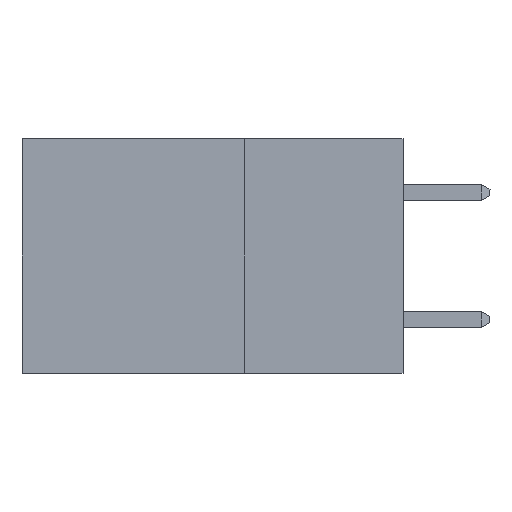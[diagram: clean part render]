
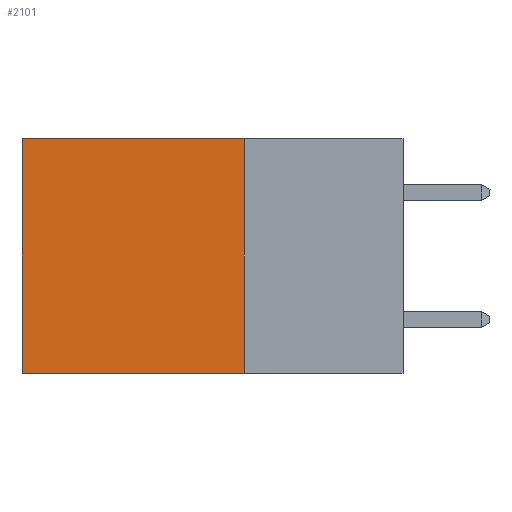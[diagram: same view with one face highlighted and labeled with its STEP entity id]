
A CAD part, left-side view. The second image highlights one B-rep face of the part: STEP entity #2101.
In plain terms, the highlighted planar face has unit normal (-1, 0, 0).
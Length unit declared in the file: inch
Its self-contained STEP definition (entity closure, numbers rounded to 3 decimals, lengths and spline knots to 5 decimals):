
#900 = ORIENTED_EDGE ( 'NONE', *, *, #17273, .T. ) ;
#932 = PLANE ( 'NONE',  #12053 ) ;
#1125 = VERTEX_POINT ( 'NONE', #2453 ) ;
#1261 = CARTESIAN_POINT ( 'NONE',  ( 0.2875, 0.25, 0. ) ) ;
#1276 = CARTESIAN_POINT ( 'NONE',  ( 0.2875, 0.25, -0.37 ) ) ;
#1285 = LINE ( 'NONE', #16964, #12396 ) ;
#1719 = DIRECTION ( 'NONE',  ( 1., 0., 0. ) ) ;
#1726 = DIRECTION ( 'NONE',  ( 0., 0., -1. ) ) ;
#2101 = ADVANCED_FACE ( 'NONE', ( #15563 ), #932, .F. ) ;
#2121 = VECTOR ( 'NONE', #16140, 39.37008 ) ;
#2247 = VERTEX_POINT ( 'NONE', #1276 ) ;
#2453 = CARTESIAN_POINT ( 'NONE',  ( 0.2875, 0.6, -0.37 ) ) ;
#3819 = LINE ( 'NONE', #8152, #14766 ) ;
#3969 = EDGE_CURVE ( 'NONE', #11564, #2247, #17895, .T. ) ;
#5431 = DIRECTION ( 'NONE',  ( 0., 1., 0. ) ) ;
#6199 = EDGE_LOOP ( 'NONE', ( #900, #13937, #10430, #12678 ) ) ;
#6577 = VECTOR ( 'NONE', #11974, 39.37008 ) ;
#7060 = DIRECTION ( 'NONE',  ( 0., 1., 0. ) ) ;
#8152 = CARTESIAN_POINT ( 'NONE',  ( 0.2875, 0.25, -0.37 ) ) ;
#9818 = LINE ( 'NONE', #14655, #2121 ) ;
#10430 = ORIENTED_EDGE ( 'NONE', *, *, #3969, .F. ) ;
#11051 = VERTEX_POINT ( 'NONE', #13479 ) ;
#11564 = VERTEX_POINT ( 'NONE', #14710 ) ;
#11974 = DIRECTION ( 'NONE',  ( 0., 0., -1. ) ) ;
#12053 = AXIS2_PLACEMENT_3D ( 'NONE', #1261, #1719, #1726 ) ;
#12396 = VECTOR ( 'NONE', #7060, 39.37008 ) ;
#12678 = ORIENTED_EDGE ( 'NONE', *, *, #13454, .T. ) ;
#13363 = CARTESIAN_POINT ( 'NONE',  ( 0.2875, 0.25, 0. ) ) ;
#13454 = EDGE_CURVE ( 'NONE', #11564, #11051, #1285, .T. ) ;
#13479 = CARTESIAN_POINT ( 'NONE',  ( 0.2875, 0.6, 0. ) ) ;
#13937 = ORIENTED_EDGE ( 'NONE', *, *, #18336, .F. ) ;
#14655 = CARTESIAN_POINT ( 'NONE',  ( 0.2875, 0.6, 0. ) ) ;
#14710 = CARTESIAN_POINT ( 'NONE',  ( 0.2875, 0.25, 0. ) ) ;
#14766 = VECTOR ( 'NONE', #5431, 39.37008 ) ;
#15563 = FACE_OUTER_BOUND ( 'NONE', #6199, .T. ) ;
#16140 = DIRECTION ( 'NONE',  ( 0., 0., -1. ) ) ;
#16964 = CARTESIAN_POINT ( 'NONE',  ( 0.2875, 0.25, 0. ) ) ;
#17273 = EDGE_CURVE ( 'NONE', #11051, #1125, #9818, .T. ) ;
#17895 = LINE ( 'NONE', #13363, #6577 ) ;
#18336 = EDGE_CURVE ( 'NONE', #2247, #1125, #3819, .T. ) ;
